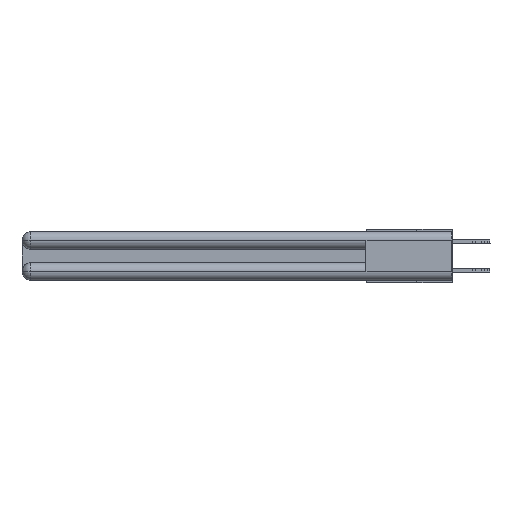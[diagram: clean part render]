
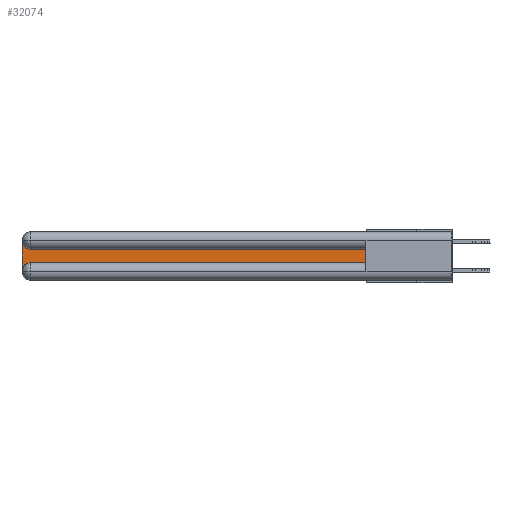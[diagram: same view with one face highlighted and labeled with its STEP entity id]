
A CAD part, left-side view. The second image highlights one B-rep face of the part: STEP entity #32074.
In plain terms, the highlighted planar face has unit normal (-1, 0, 0).
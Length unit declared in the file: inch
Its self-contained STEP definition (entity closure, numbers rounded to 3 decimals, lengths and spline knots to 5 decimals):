
#910 = EDGE_CURVE ( 'NONE', #29961, #17035, #19133, .T. ) ;
#2454 = ORIENTED_EDGE ( 'NONE', *, *, #910, .T. ) ;
#2556 = DIRECTION ( 'NONE',  ( 0., 0., -1. ) ) ;
#3211 = AXIS2_PLACEMENT_3D ( 'NONE', #3449, #8576, #22104 ) ;
#3449 = CARTESIAN_POINT ( 'NONE',  ( 0.075, 2.94, -0.2775 ) ) ;
#3974 = DIRECTION ( 'NONE',  ( 0., 1., 0. ) ) ;
#4186 = CARTESIAN_POINT ( 'NONE',  ( 0.075, 0.6, -0.2175 ) ) ;
#4390 = CARTESIAN_POINT ( 'NONE',  ( 0.075, 0.6, -0.2175 ) ) ;
#4731 = VERTEX_POINT ( 'NONE', #29358 ) ;
#4930 = VECTOR ( 'NONE', #3974, 39.37008 ) ;
#5340 = ORIENTED_EDGE ( 'NONE', *, *, #9352, .T. ) ;
#5567 = EDGE_CURVE ( 'NONE', #27383, #29961, #32477, .T. ) ;
#8576 = DIRECTION ( 'NONE',  ( 1., 0., 0. ) ) ;
#9352 = EDGE_CURVE ( 'NONE', #17035, #34131, #21852, .T. ) ;
#9411 = DIRECTION ( 'NONE',  ( 0., 0., -1. ) ) ;
#9816 = AXIS2_PLACEMENT_3D ( 'NONE', #31372, #10083, #34409 ) ;
#10083 = DIRECTION ( 'NONE',  ( 1., 0., 0. ) ) ;
#10314 = CARTESIAN_POINT ( 'NONE',  ( 0.075, 0.6, -0.1225 ) ) ;
#10943 = CARTESIAN_POINT ( 'NONE',  ( 0.075, 3., -0.2175 ) ) ;
#11445 = EDGE_LOOP ( 'NONE', ( #2454, #5340, #16974, #32007, #19700, #29339 ) ) ;
#12566 = CIRCLE ( 'NONE', #3211, 0.06 ) ;
#13293 = EDGE_CURVE ( 'NONE', #4731, #13914, #12566, .T. ) ;
#13914 = VERTEX_POINT ( 'NONE', #19843 ) ;
#14278 = DIRECTION ( 'NONE',  ( 1., 0., 0. ) ) ;
#14571 = CARTESIAN_POINT ( 'NONE',  ( 0.075, 0.6, -0.1225 ) ) ;
#15748 = CARTESIAN_POINT ( 'NONE',  ( 0.075, 3., -0.0625 ) ) ;
#16974 = ORIENTED_EDGE ( 'NONE', *, *, #20100, .T. ) ;
#17035 = VERTEX_POINT ( 'NONE', #27919 ) ;
#17207 = PLANE ( 'NONE',  #22327 ) ;
#18699 = EDGE_CURVE ( 'NONE', #13914, #27383, #29500, .T. ) ;
#19133 = LINE ( 'NONE', #14571, #4930 ) ;
#19700 = ORIENTED_EDGE ( 'NONE', *, *, #18699, .T. ) ;
#19843 = CARTESIAN_POINT ( 'NONE',  ( 0.075, 2.94, -0.2175 ) ) ;
#20100 = EDGE_CURVE ( 'NONE', #34131, #4731, #33605, .T. ) ;
#21852 = CIRCLE ( 'NONE', #9816, 0.06 ) ;
#22104 = DIRECTION ( 'NONE',  ( 0., 0., -1. ) ) ;
#22327 = AXIS2_PLACEMENT_3D ( 'NONE', #27904, #14278, #9411 ) ;
#22435 = VECTOR ( 'NONE', #33980, 39.37008 ) ;
#24638 = FACE_OUTER_BOUND ( 'NONE', #11445, .T. ) ;
#25160 = DIRECTION ( 'NONE',  ( 0., 0., 1. ) ) ;
#27120 = VECTOR ( 'NONE', #25160, 39.37008 ) ;
#27383 = VERTEX_POINT ( 'NONE', #4186 ) ;
#27904 = CARTESIAN_POINT ( 'NONE',  ( 0.075, 3., -0.1225 ) ) ;
#27919 = CARTESIAN_POINT ( 'NONE',  ( 0.075, 2.94, -0.1225 ) ) ;
#28168 = VECTOR ( 'NONE', #2556, 39.37008 ) ;
#29339 = ORIENTED_EDGE ( 'NONE', *, *, #5567, .T. ) ;
#29358 = CARTESIAN_POINT ( 'NONE',  ( 0.075, 3., -0.2775 ) ) ;
#29500 = LINE ( 'NONE', #4390, #22435 ) ;
#29961 = VERTEX_POINT ( 'NONE', #10314 ) ;
#31372 = CARTESIAN_POINT ( 'NONE',  ( 0.075, 2.94, -0.0625 ) ) ;
#32007 = ORIENTED_EDGE ( 'NONE', *, *, #13293, .T. ) ;
#32074 = ADVANCED_FACE ( 'NONE', ( #24638 ), #17207, .F. ) ;
#32477 = LINE ( 'NONE', #33047, #27120 ) ;
#33047 = CARTESIAN_POINT ( 'NONE',  ( 0.075, 0.6, -0.2175 ) ) ;
#33605 = LINE ( 'NONE', #10943, #28168 ) ;
#33980 = DIRECTION ( 'NONE',  ( 0., -1., 0. ) ) ;
#34131 = VERTEX_POINT ( 'NONE', #15748 ) ;
#34409 = DIRECTION ( 'NONE',  ( 0., 0., -1. ) ) ;
